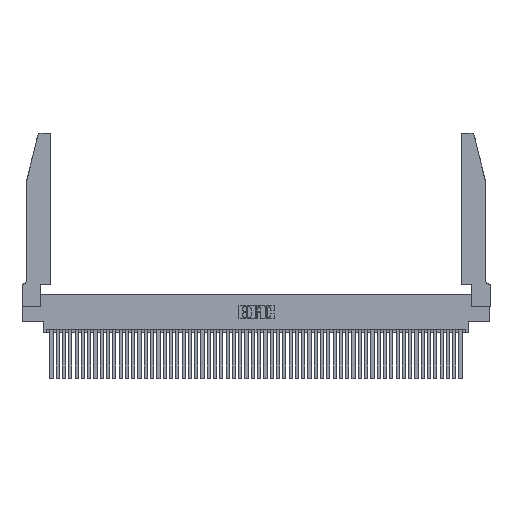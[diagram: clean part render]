
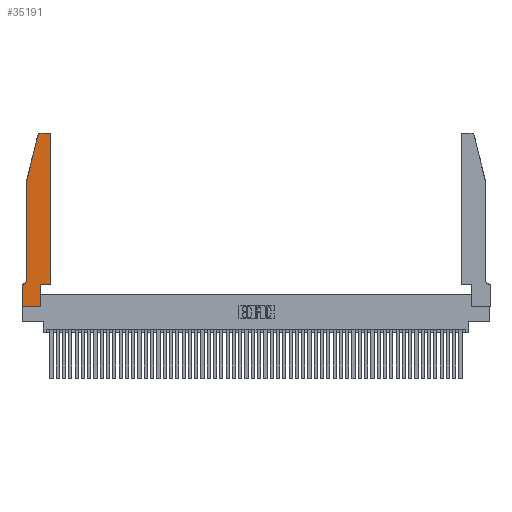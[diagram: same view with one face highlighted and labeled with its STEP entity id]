
A CAD part, top view. The second image highlights one B-rep face of the part: STEP entity #35191.
In plain terms, the highlighted planar face has unit normal (0, 0, 1).
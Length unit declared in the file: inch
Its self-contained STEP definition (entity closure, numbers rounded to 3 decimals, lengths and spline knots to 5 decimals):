
#13 = ORIENTED_EDGE ( 'NONE', *, *, #34366, .T. ) ;
#139 = VERTEX_POINT ( 'NONE', #48797 ) ;
#287 = DIRECTION ( 'NONE',  ( 1., 0., 0. ) ) ;
#357 = CARTESIAN_POINT ( 'NONE',  ( 0.0755, 0.35, 0.37 ) ) ;
#869 = LINE ( 'NONE', #27047, #20170 ) ;
#1307 = EDGE_CURVE ( 'NONE', #17330, #45817, #26786, .T. ) ;
#1938 = CARTESIAN_POINT ( 'NONE',  ( 0.2865, 0., 0.37 ) ) ;
#2214 = PLANE ( 'NONE',  #16575 ) ;
#2610 = LINE ( 'NONE', #36957, #28957 ) ;
#3145 = AXIS2_PLACEMENT_3D ( 'NONE', #47405, #18247, #34596 ) ;
#3389 = LINE ( 'NONE', #19424, #51021 ) ;
#3587 = EDGE_CURVE ( 'NONE', #47883, #41746, #17496, .T. ) ;
#3595 = ORIENTED_EDGE ( 'NONE', *, *, #40837, .T. ) ;
#3788 = VECTOR ( 'NONE', #29490, 39.37008 ) ;
#5286 = ORIENTED_EDGE ( 'NONE', *, *, #17468, .T. ) ;
#5350 = VECTOR ( 'NONE', #9689, 39.37008 ) ;
#6535 = ORIENTED_EDGE ( 'NONE', *, *, #36501, .T. ) ;
#7031 = CARTESIAN_POINT ( 'NONE',  ( 0.2865, 0.35, 0.37 ) ) ;
#7803 = CARTESIAN_POINT ( 'NONE',  ( 0.2605, 2.75, 0.37 ) ) ;
#8225 = EDGE_LOOP ( 'NONE', ( #23157, #20847, #20920, #44627, #13, #18333, #32613, #3595, #12124, #6535, #5286, #16080 ) ) ;
#9540 = LINE ( 'NONE', #357, #3788 ) ;
#9689 = DIRECTION ( 'NONE',  ( 0., 1., 0. ) ) ;
#11519 = CARTESIAN_POINT ( 'NONE',  ( 0., 0.35, 0.37 ) ) ;
#12124 = ORIENTED_EDGE ( 'NONE', *, *, #23584, .T. ) ;
#12501 = LINE ( 'NONE', #7803, #51127 ) ;
#13332 = LINE ( 'NONE', #27863, #50707 ) ;
#13342 = VERTEX_POINT ( 'NONE', #32449 ) ;
#13993 = VERTEX_POINT ( 'NONE', #7031 ) ;
#16080 = ORIENTED_EDGE ( 'NONE', *, *, #3587, .T. ) ;
#16575 = AXIS2_PLACEMENT_3D ( 'NONE', #11519, #19787, #35079 ) ;
#16777 = EDGE_CURVE ( 'NONE', #41746, #28233, #12501, .T. ) ;
#17302 = VECTOR ( 'NONE', #30406, 39.37008 ) ;
#17330 = VERTEX_POINT ( 'NONE', #25163 ) ;
#17468 = EDGE_CURVE ( 'NONE', #40775, #47883, #18842, .T. ) ;
#17496 = CIRCLE ( 'NONE', #50039, 0.03 ) ;
#18247 = DIRECTION ( 'NONE',  ( 0., 0., -1. ) ) ;
#18333 = ORIENTED_EDGE ( 'NONE', *, *, #48792, .T. ) ;
#18842 = LINE ( 'NONE', #33973, #5350 ) ;
#19424 = CARTESIAN_POINT ( 'NONE',  ( 0., 0., 0.37 ) ) ;
#19787 = DIRECTION ( 'NONE',  ( 0., 0., 1. ) ) ;
#20170 = VECTOR ( 'NONE', #27396, 39.37008 ) ;
#20472 = EDGE_CURVE ( 'NONE', #33379, #17330, #27601, .T. ) ;
#20595 = CARTESIAN_POINT ( 'NONE',  ( 0.284, 2.72, 0.37 ) ) ;
#20847 = ORIENTED_EDGE ( 'NONE', *, *, #42393, .T. ) ;
#20920 = ORIENTED_EDGE ( 'NONE', *, *, #20472, .T. ) ;
#21027 = CARTESIAN_POINT ( 'NONE',  ( 0.0755, 0.42, 0.37 ) ) ;
#22436 = DIRECTION ( 'NONE',  ( 0., 0., 1. ) ) ;
#22612 = CARTESIAN_POINT ( 'NONE',  ( 0.4205, 2.72, 0.37 ) ) ;
#22887 = VECTOR ( 'NONE', #27795, 39.37008 ) ;
#23157 = ORIENTED_EDGE ( 'NONE', *, *, #16777, .T. ) ;
#23584 = EDGE_CURVE ( 'NONE', #25035, #13993, #13332, .T. ) ;
#24930 = DIRECTION ( 'NONE',  ( 1., 0., 0. ) ) ;
#24993 = CARTESIAN_POINT ( 'NONE',  ( 0., 0.35, 0.37 ) ) ;
#25035 = VERTEX_POINT ( 'NONE', #1938 ) ;
#25163 = CARTESIAN_POINT ( 'NONE',  ( 0.0755, 2., 0.37 ) ) ;
#25997 = EDGE_CURVE ( 'NONE', #26317, #13342, #3389, .T. ) ;
#26317 = VERTEX_POINT ( 'NONE', #24993 ) ;
#26786 = LINE ( 'NONE', #35702, #22887 ) ;
#27047 = CARTESIAN_POINT ( 'NONE',  ( 0., 0., 0.37 ) ) ;
#27396 = DIRECTION ( 'NONE',  ( 1., 0., 0. ) ) ;
#27601 = LINE ( 'NONE', #46822, #17302 ) ;
#27795 = DIRECTION ( 'NONE',  ( 0., -1., 0. ) ) ;
#27863 = CARTESIAN_POINT ( 'NONE',  ( 0.2865, 0.35, 0.37 ) ) ;
#28233 = VERTEX_POINT ( 'NONE', #29614 ) ;
#28957 = VECTOR ( 'NONE', #24930, 39.37008 ) ;
#29490 = DIRECTION ( 'NONE',  ( -1., 0., 0. ) ) ;
#29614 = CARTESIAN_POINT ( 'NONE',  ( 0.284, 2.75, 0.37 ) ) ;
#30406 = DIRECTION ( 'NONE',  ( -0.239, -0.971, 0. ) ) ;
#31672 = DIRECTION ( 'NONE',  ( 0., -1., 0. ) ) ;
#32449 = CARTESIAN_POINT ( 'NONE',  ( 0., 0., 0.37 ) ) ;
#32613 = ORIENTED_EDGE ( 'NONE', *, *, #25997, .T. ) ;
#33379 = VERTEX_POINT ( 'NONE', #48576 ) ;
#33777 = CIRCLE ( 'NONE', #3145, 0.07 ) ;
#33973 = CARTESIAN_POINT ( 'NONE',  ( 0.4505, 0.35, 0.37 ) ) ;
#34366 = EDGE_CURVE ( 'NONE', #45817, #139, #33777, .T. ) ;
#34596 = DIRECTION ( 'NONE',  ( -1., 0., 0. ) ) ;
#35079 = DIRECTION ( 'NONE',  ( 1., 0., 0. ) ) ;
#35191 = ADVANCED_FACE ( 'NONE', ( #49084 ), #2214, .T. ) ;
#35702 = CARTESIAN_POINT ( 'NONE',  ( 0.0755, 2., 0.37 ) ) ;
#36501 = EDGE_CURVE ( 'NONE', #13993, #40775, #2610, .T. ) ;
#36957 = CARTESIAN_POINT ( 'NONE',  ( 0.4505, 0.35, 0.37 ) ) ;
#37587 = CARTESIAN_POINT ( 'NONE',  ( 0.4505, 2.72, 0.37 ) ) ;
#37793 = DIRECTION ( 'NONE',  ( -1., 0., 0. ) ) ;
#38808 = DIRECTION ( 'NONE',  ( 1., 0., 0. ) ) ;
#40775 = VERTEX_POINT ( 'NONE', #42526 ) ;
#40837 = EDGE_CURVE ( 'NONE', #13342, #25035, #869, .T. ) ;
#41681 = CARTESIAN_POINT ( 'NONE',  ( 0.4205, 2.75, 0.37 ) ) ;
#41746 = VERTEX_POINT ( 'NONE', #41681 ) ;
#42393 = EDGE_CURVE ( 'NONE', #28233, #33379, #44175, .T. ) ;
#42526 = CARTESIAN_POINT ( 'NONE',  ( 0.4505, 0.35, 0.37 ) ) ;
#44175 = CIRCLE ( 'NONE', #51260, 0.03 ) ;
#44627 = ORIENTED_EDGE ( 'NONE', *, *, #1307, .T. ) ;
#45817 = VERTEX_POINT ( 'NONE', #21027 ) ;
#46822 = CARTESIAN_POINT ( 'NONE',  ( 0.0755, 2., 0.37 ) ) ;
#47405 = CARTESIAN_POINT ( 'NONE',  ( 0.0055, 0.42, 0.37 ) ) ;
#47883 = VERTEX_POINT ( 'NONE', #37587 ) ;
#48576 = CARTESIAN_POINT ( 'NONE',  ( 0.25487, 2.72718, 0.37 ) ) ;
#48792 = EDGE_CURVE ( 'NONE', #139, #26317, #9540, .T. ) ;
#48797 = CARTESIAN_POINT ( 'NONE',  ( 0.0055, 0.35, 0.37 ) ) ;
#49084 = FACE_OUTER_BOUND ( 'NONE', #8225, .T. ) ;
#49394 = DIRECTION ( 'NONE',  ( 0., 0., 1. ) ) ;
#50039 = AXIS2_PLACEMENT_3D ( 'NONE', #22612, #22436, #38808 ) ;
#50707 = VECTOR ( 'NONE', #51964, 39.37008 ) ;
#51021 = VECTOR ( 'NONE', #31672, 39.37008 ) ;
#51127 = VECTOR ( 'NONE', #37793, 39.37008 ) ;
#51260 = AXIS2_PLACEMENT_3D ( 'NONE', #20595, #49394, #287 ) ;
#51964 = DIRECTION ( 'NONE',  ( 0., 1., 0. ) ) ;
